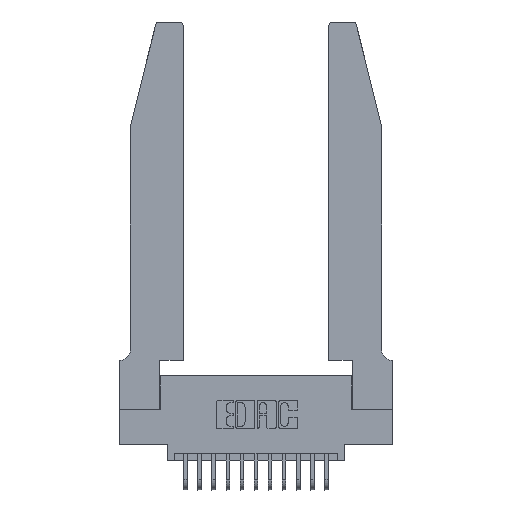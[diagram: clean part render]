
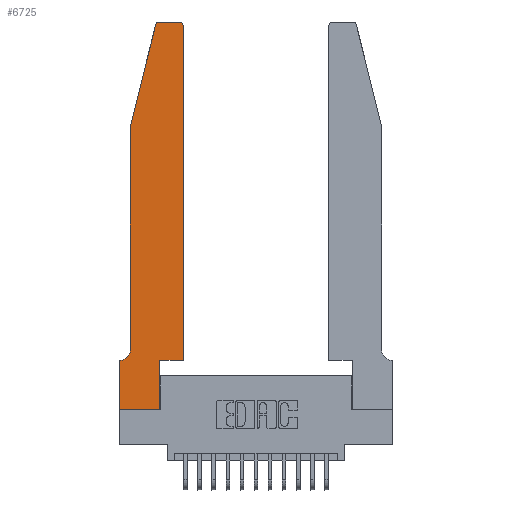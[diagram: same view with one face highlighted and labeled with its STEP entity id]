
A CAD part, top view. The second image highlights one B-rep face of the part: STEP entity #6725.
In plain terms, the highlighted planar face has unit normal (0, 0, 1).
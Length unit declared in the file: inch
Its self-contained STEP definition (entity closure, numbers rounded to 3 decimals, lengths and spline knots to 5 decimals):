
#130 = CARTESIAN_POINT ( 'NONE',  ( 0., 0.35, 0.37 ) ) ;
#217 = EDGE_CURVE ( 'NONE', #4666, #13918, #10479, .T. ) ;
#226 = CARTESIAN_POINT ( 'NONE',  ( 0.0055, 0.42, 0.37 ) ) ;
#434 = VERTEX_POINT ( 'NONE', #5313 ) ;
#508 = CARTESIAN_POINT ( 'NONE',  ( 0.0755, 0.35, 0.37 ) ) ;
#750 = CARTESIAN_POINT ( 'NONE',  ( 0.4505, 0.35, 0.37 ) ) ;
#946 = EDGE_CURVE ( 'NONE', #434, #6083, #10396, .T. ) ;
#1052 = CARTESIAN_POINT ( 'NONE',  ( 0., 0., 0.37 ) ) ;
#1105 = DIRECTION ( 'NONE',  ( 0., -1., 0. ) ) ;
#1173 = CARTESIAN_POINT ( 'NONE',  ( 0.2865, 0.35, 0.37 ) ) ;
#1374 = LINE ( 'NONE', #1173, #17291 ) ;
#1416 = CIRCLE ( 'NONE', #12022, 0.03 ) ;
#1525 = VECTOR ( 'NONE', #18540, 39.37008 ) ;
#1652 = PLANE ( 'NONE',  #10648 ) ;
#1746 = DIRECTION ( 'NONE',  ( -1., 0., 0. ) ) ;
#1782 = VECTOR ( 'NONE', #6436, 39.37008 ) ;
#2306 = DIRECTION ( 'NONE',  ( -0.239, -0.971, 0. ) ) ;
#2334 = VECTOR ( 'NONE', #4074, 39.37008 ) ;
#2487 = EDGE_CURVE ( 'NONE', #6083, #7363, #4466, .T. ) ;
#2551 = DIRECTION ( 'NONE',  ( 1., 0., 0. ) ) ;
#2621 = CARTESIAN_POINT ( 'NONE',  ( 0.4505, 0.35, 0.37 ) ) ;
#2658 = ORIENTED_EDGE ( 'NONE', *, *, #946, .T. ) ;
#2766 = CIRCLE ( 'NONE', #4668, 0.03 ) ;
#2799 = CARTESIAN_POINT ( 'NONE',  ( 0.4505, 0.35, 0.37 ) ) ;
#2998 = VERTEX_POINT ( 'NONE', #10637 ) ;
#3134 = DIRECTION ( 'NONE',  ( 0., 0., 1. ) ) ;
#3512 = VERTEX_POINT ( 'NONE', #11593 ) ;
#3581 = ORIENTED_EDGE ( 'NONE', *, *, #12543, .T. ) ;
#3699 = ORIENTED_EDGE ( 'NONE', *, *, #8352, .T. ) ;
#3786 = ORIENTED_EDGE ( 'NONE', *, *, #2487, .T. ) ;
#3873 = EDGE_CURVE ( 'NONE', #7120, #434, #1416, .T. ) ;
#3951 = CARTESIAN_POINT ( 'NONE',  ( 0.284, 2.75, 0.37 ) ) ;
#3960 = ORIENTED_EDGE ( 'NONE', *, *, #15962, .T. ) ;
#4074 = DIRECTION ( 'NONE',  ( 0., 1., 0. ) ) ;
#4379 = ORIENTED_EDGE ( 'NONE', *, *, #217, .T. ) ;
#4466 = LINE ( 'NONE', #8301, #7974 ) ;
#4613 = CARTESIAN_POINT ( 'NONE',  ( 0., 0., 0.37 ) ) ;
#4622 = CARTESIAN_POINT ( 'NONE',  ( 0.0755, 2., 0.37 ) ) ;
#4666 = VERTEX_POINT ( 'NONE', #12644 ) ;
#4668 = AXIS2_PLACEMENT_3D ( 'NONE', #16583, #7585, #18100 ) ;
#5258 = CARTESIAN_POINT ( 'NONE',  ( 0.284, 2.72, 0.37 ) ) ;
#5313 = CARTESIAN_POINT ( 'NONE',  ( 0.25487, 2.72718, 0.37 ) ) ;
#5442 = LINE ( 'NONE', #17023, #1525 ) ;
#5960 = FACE_OUTER_BOUND ( 'NONE', #13933, .T. ) ;
#6083 = VERTEX_POINT ( 'NONE', #4622 ) ;
#6112 = DIRECTION ( 'NONE',  ( 0., -1., 0. ) ) ;
#6273 = VECTOR ( 'NONE', #2551, 39.37008 ) ;
#6350 = CARTESIAN_POINT ( 'NONE',  ( 0.4505, 2.72, 0.37 ) ) ;
#6436 = DIRECTION ( 'NONE',  ( -1., 0., 0. ) ) ;
#6725 = ADVANCED_FACE ( 'NONE', ( #5960 ), #1652, .T. ) ;
#6750 = LINE ( 'NONE', #2621, #2334 ) ;
#7120 = VERTEX_POINT ( 'NONE', #3951 ) ;
#7308 = CARTESIAN_POINT ( 'NONE',  ( 0., 0.35, 0.37 ) ) ;
#7349 = LINE ( 'NONE', #4613, #18836 ) ;
#7363 = VERTEX_POINT ( 'NONE', #7548 ) ;
#7548 = CARTESIAN_POINT ( 'NONE',  ( 0.0755, 0.42, 0.37 ) ) ;
#7585 = DIRECTION ( 'NONE',  ( 0., 0., 1. ) ) ;
#7974 = VECTOR ( 'NONE', #1105, 39.37008 ) ;
#8301 = CARTESIAN_POINT ( 'NONE',  ( 0.0755, 2., 0.37 ) ) ;
#8352 = EDGE_CURVE ( 'NONE', #13918, #16013, #7349, .T. ) ;
#8500 = EDGE_CURVE ( 'NONE', #3512, #7120, #5442, .T. ) ;
#9211 = CARTESIAN_POINT ( 'NONE',  ( 0., 0., 0.37 ) ) ;
#10396 = LINE ( 'NONE', #15392, #13925 ) ;
#10479 = LINE ( 'NONE', #508, #1782 ) ;
#10522 = ORIENTED_EDGE ( 'NONE', *, *, #3873, .T. ) ;
#10637 = CARTESIAN_POINT ( 'NONE',  ( 0.2865, 0.35, 0.37 ) ) ;
#10648 = AXIS2_PLACEMENT_3D ( 'NONE', #130, #3134, #13620 ) ;
#10666 = DIRECTION ( 'NONE',  ( 0., 0., -1. ) ) ;
#11274 = CIRCLE ( 'NONE', #12521, 0.07 ) ;
#11424 = VECTOR ( 'NONE', #14793, 39.37008 ) ;
#11464 = ORIENTED_EDGE ( 'NONE', *, *, #12485, .T. ) ;
#11593 = CARTESIAN_POINT ( 'NONE',  ( 0.4205, 2.75, 0.37 ) ) ;
#11657 = CARTESIAN_POINT ( 'NONE',  ( 0.2865, 0., 0.37 ) ) ;
#12022 = AXIS2_PLACEMENT_3D ( 'NONE', #5258, #17336, #15744 ) ;
#12257 = VERTEX_POINT ( 'NONE', #6350 ) ;
#12446 = ORIENTED_EDGE ( 'NONE', *, *, #16872, .T. ) ;
#12485 = EDGE_CURVE ( 'NONE', #16919, #2998, #1374, .T. ) ;
#12521 = AXIS2_PLACEMENT_3D ( 'NONE', #226, #10666, #1746 ) ;
#12543 = EDGE_CURVE ( 'NONE', #2998, #19189, #15879, .T. ) ;
#12644 = CARTESIAN_POINT ( 'NONE',  ( 0.0055, 0.35, 0.37 ) ) ;
#13088 = DIRECTION ( 'NONE',  ( 0., 1., 0. ) ) ;
#13620 = DIRECTION ( 'NONE',  ( 1., 0., 0. ) ) ;
#13918 = VERTEX_POINT ( 'NONE', #7308 ) ;
#13925 = VECTOR ( 'NONE', #2306, 39.37008 ) ;
#13933 = EDGE_LOOP ( 'NONE', ( #16372, #10522, #2658, #3786, #3960, #4379, #3699, #12446, #11464, #3581, #18215, #18492 ) ) ;
#14773 = LINE ( 'NONE', #1052, #6273 ) ;
#14793 = DIRECTION ( 'NONE',  ( 1., 0., 0. ) ) ;
#15392 = CARTESIAN_POINT ( 'NONE',  ( 0.0755, 2., 0.37 ) ) ;
#15744 = DIRECTION ( 'NONE',  ( 1., 0., 0. ) ) ;
#15879 = LINE ( 'NONE', #2799, #11424 ) ;
#15962 = EDGE_CURVE ( 'NONE', #7363, #4666, #11274, .T. ) ;
#16013 = VERTEX_POINT ( 'NONE', #9211 ) ;
#16372 = ORIENTED_EDGE ( 'NONE', *, *, #8500, .T. ) ;
#16583 = CARTESIAN_POINT ( 'NONE',  ( 0.4205, 2.72, 0.37 ) ) ;
#16872 = EDGE_CURVE ( 'NONE', #16013, #16919, #14773, .T. ) ;
#16902 = EDGE_CURVE ( 'NONE', #19189, #12257, #6750, .T. ) ;
#16919 = VERTEX_POINT ( 'NONE', #11657 ) ;
#17023 = CARTESIAN_POINT ( 'NONE',  ( 0.2605, 2.75, 0.37 ) ) ;
#17291 = VECTOR ( 'NONE', #13088, 39.37008 ) ;
#17336 = DIRECTION ( 'NONE',  ( 0., 0., 1. ) ) ;
#18100 = DIRECTION ( 'NONE',  ( 1., 0., 0. ) ) ;
#18215 = ORIENTED_EDGE ( 'NONE', *, *, #16902, .T. ) ;
#18492 = ORIENTED_EDGE ( 'NONE', *, *, #18956, .T. ) ;
#18540 = DIRECTION ( 'NONE',  ( -1., 0., 0. ) ) ;
#18836 = VECTOR ( 'NONE', #6112, 39.37008 ) ;
#18956 = EDGE_CURVE ( 'NONE', #12257, #3512, #2766, .T. ) ;
#19189 = VERTEX_POINT ( 'NONE', #750 ) ;
